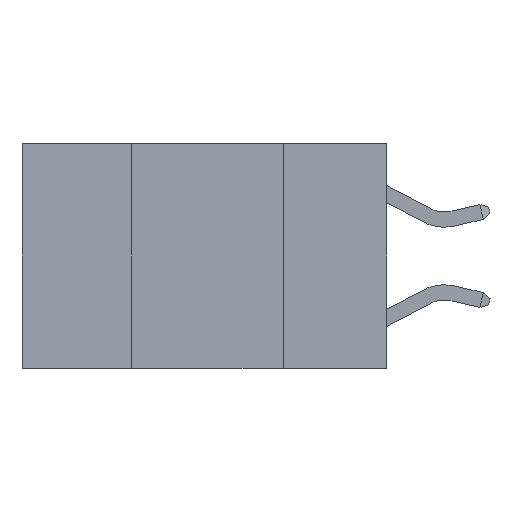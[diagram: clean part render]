
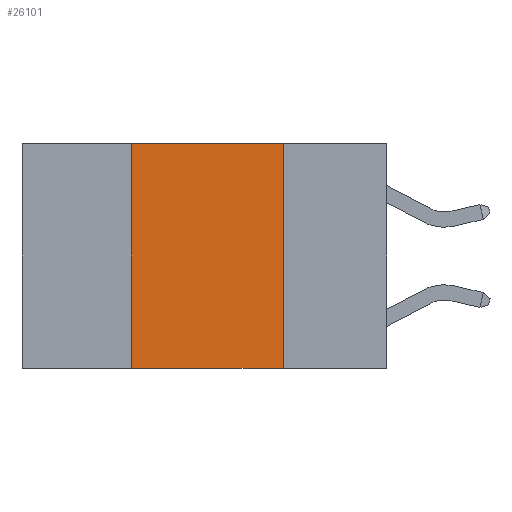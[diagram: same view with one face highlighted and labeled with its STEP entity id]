
A CAD part, left-side view. The second image highlights one B-rep face of the part: STEP entity #26101.
In plain terms, the highlighted planar face has unit normal (-1, 0, 0).
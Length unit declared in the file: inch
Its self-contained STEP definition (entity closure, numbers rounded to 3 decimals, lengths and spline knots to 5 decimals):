
#418 = AXIS2_PLACEMENT_3D ( 'NONE', #16316, #3907, #18407 ) ;
#500 = CARTESIAN_POINT ( 'NONE',  ( 0., 0.42, 0. ) ) ;
#1074 = LINE ( 'NONE', #22567, #17698 ) ;
#1168 = CARTESIAN_POINT ( 'NONE',  ( 0., 0.6, 0. ) ) ;
#1643 = CARTESIAN_POINT ( 'NONE',  ( 0., 0.17, 0. ) ) ;
#1740 = PLANE ( 'NONE',  #418 ) ;
#1933 = CARTESIAN_POINT ( 'NONE',  ( 0., 0.42, 0. ) ) ;
#3326 = VERTEX_POINT ( 'NONE', #12227 ) ;
#3841 = EDGE_CURVE ( 'NONE', #19002, #14499, #11287, .T. ) ;
#3907 = DIRECTION ( 'NONE',  ( 1., 0., 0. ) ) ;
#4668 = VECTOR ( 'NONE', #26344, 39.37008 ) ;
#5714 = VECTOR ( 'NONE', #13706, 39.37008 ) ;
#5788 = EDGE_CURVE ( 'NONE', #3326, #7100, #10243, .T. ) ;
#6194 = ORIENTED_EDGE ( 'NONE', *, *, #5788, .T. ) ;
#6213 = DIRECTION ( 'NONE',  ( 0., 0., 1. ) ) ;
#7100 = VERTEX_POINT ( 'NONE', #22458 ) ;
#10005 = CARTESIAN_POINT ( 'NONE',  ( 0., 0.6, -0.37 ) ) ;
#10243 = LINE ( 'NONE', #10005, #4668 ) ;
#10332 = DIRECTION ( 'NONE',  ( 0., 0., -1. ) ) ;
#11287 = LINE ( 'NONE', #1168, #5714 ) ;
#11753 = ORIENTED_EDGE ( 'NONE', *, *, #17969, .F. ) ;
#12227 = CARTESIAN_POINT ( 'NONE',  ( 0., 0.42, -0.37 ) ) ;
#12937 = EDGE_LOOP ( 'NONE', ( #23533, #23887, #11753, #6194 ) ) ;
#13706 = DIRECTION ( 'NONE',  ( 0., -1., 0. ) ) ;
#14499 = VERTEX_POINT ( 'NONE', #1643 ) ;
#16316 = CARTESIAN_POINT ( 'NONE',  ( 0., 0.6, 0. ) ) ;
#17698 = VECTOR ( 'NONE', #10332, 39.37008 ) ;
#17969 = EDGE_CURVE ( 'NONE', #3326, #19002, #24913, .T. ) ;
#18407 = DIRECTION ( 'NONE',  ( 0., 0., -1. ) ) ;
#19002 = VERTEX_POINT ( 'NONE', #500 ) ;
#19512 = VECTOR ( 'NONE', #6213, 39.37008 ) ;
#22458 = CARTESIAN_POINT ( 'NONE',  ( 0., 0.17, -0.37 ) ) ;
#22567 = CARTESIAN_POINT ( 'NONE',  ( 0., 0.17, 0. ) ) ;
#23533 = ORIENTED_EDGE ( 'NONE', *, *, #26135, .F. ) ;
#23739 = FACE_OUTER_BOUND ( 'NONE', #12937, .T. ) ;
#23887 = ORIENTED_EDGE ( 'NONE', *, *, #3841, .F. ) ;
#24913 = LINE ( 'NONE', #1933, #19512 ) ;
#26101 = ADVANCED_FACE ( 'NONE', ( #23739 ), #1740, .F. ) ;
#26135 = EDGE_CURVE ( 'NONE', #14499, #7100, #1074, .T. ) ;
#26344 = DIRECTION ( 'NONE',  ( 0., -1., 0. ) ) ;
